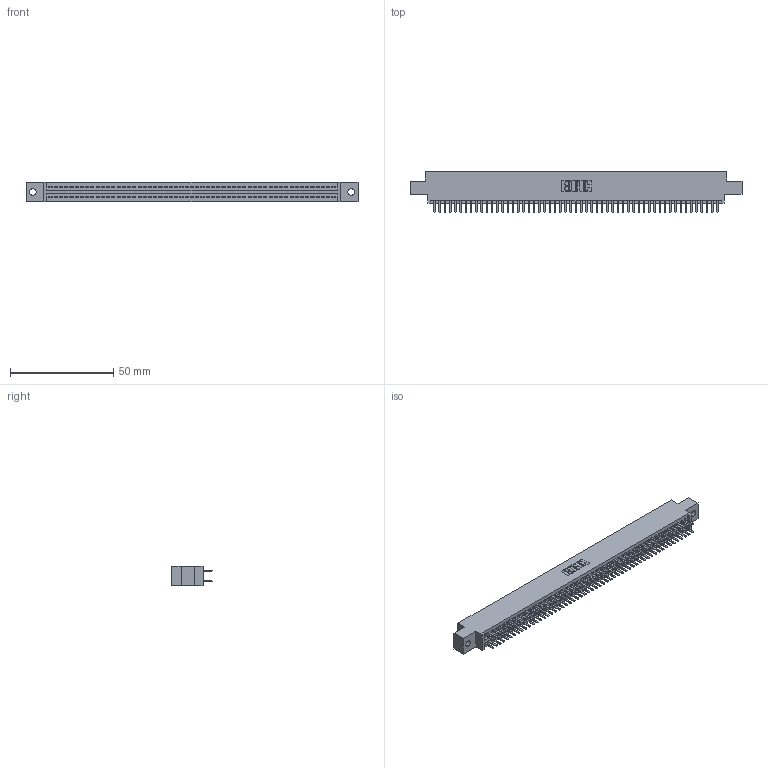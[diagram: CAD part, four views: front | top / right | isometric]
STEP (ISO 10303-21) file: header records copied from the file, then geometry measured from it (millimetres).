
FILE_DESCRIPTION (( 'STEP AP203' ), '1' );
FILE_NAME ('395-110-520-802.STEP', '2018-12-01T01:22:42', ( '' ), ( '' ), 'SwSTEP 2.0', 'SolidWorks 2016', '' );
FILE_SCHEMA (( 'CONFIG_CONTROL_DESIGN' ));
Length unit declared in the file: inch
Products named in the file (3): 395-110-520-802; 345 Part_0.170 Offset - 0.128 Dia; 345-292-001_345-293-120
Assembly tree (111 placements, depth 2):
  395-110-520-802
    345 Part_0.170 Offset - 0.128 Dia
    345-292-001_345-293-120  x110
Bounding box: 160.91 x 19.68 x 9.4 mm (x, y, z)
Volume: 15553.1 mm3; surface area: 23009.8 mm2
Topology: 111 solids, 111 shells, 6070 faces, 17623 edges, 11454 vertices
Faces by surface type: plane 3934, cylinder 2136
Entity records: 41653 total; most frequent: CARTESIAN_POINT 6984, ORIENTED_EDGE 6906, DIRECTION 6129, EDGE_CURVE 3453, LINE 3097, VECTOR 3097, VERTEX_POINT 2298, AXIS2_PLACEMENT_3D 1516
